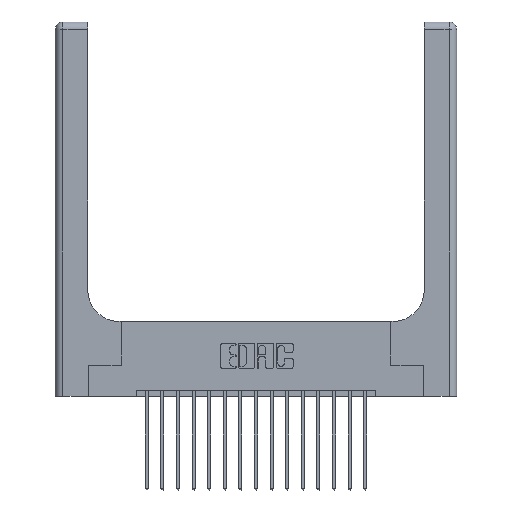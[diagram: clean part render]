
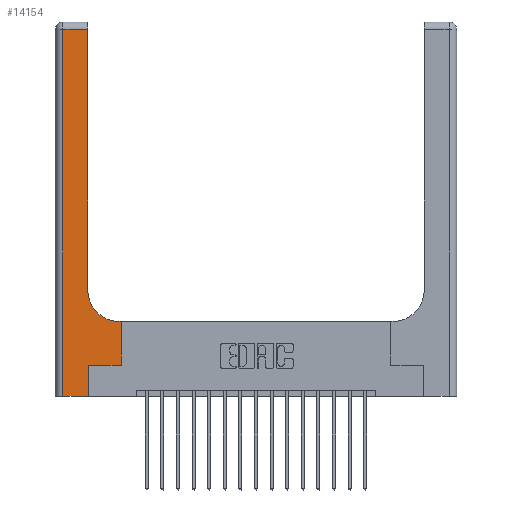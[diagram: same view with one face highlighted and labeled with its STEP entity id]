
A CAD part, top view. The second image highlights one B-rep face of the part: STEP entity #14154.
In plain terms, the highlighted planar face has unit normal (0, 0, 1).
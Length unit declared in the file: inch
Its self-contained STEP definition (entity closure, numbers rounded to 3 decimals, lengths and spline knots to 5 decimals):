
#141 = LINE ( 'NONE', #2446, #17210 ) ;
#380 = PLANE ( 'NONE',  #745 ) ;
#745 = AXIS2_PLACEMENT_3D ( 'NONE', #10289, #16165, #10420 ) ;
#1096 = VECTOR ( 'NONE', #14397, 39.37008 ) ;
#2202 = ORIENTED_EDGE ( 'NONE', *, *, #16690, .T. ) ;
#2215 = LINE ( 'NONE', #14594, #1096 ) ;
#2264 = EDGE_CURVE ( 'NONE', #12493, #14956, #2215, .T. ) ;
#2284 = VECTOR ( 'NONE', #2603, 39.37008 ) ;
#2409 = CARTESIAN_POINT ( 'NONE',  ( 0., 0., 0.37 ) ) ;
#2446 = CARTESIAN_POINT ( 'NONE',  ( 0.26, 0.6, 0.37 ) ) ;
#2603 = DIRECTION ( 'NONE',  ( -1., 0., 0. ) ) ;
#2805 = CARTESIAN_POINT ( 'NONE',  ( 0.26, 0.85, 0.37 ) ) ;
#2861 = DIRECTION ( 'NONE',  ( 0., 1., 0. ) ) ;
#3037 = FACE_OUTER_BOUND ( 'NONE', #11955, .T. ) ;
#3097 = VERTEX_POINT ( 'NONE', #7865 ) ;
#3515 = ORIENTED_EDGE ( 'NONE', *, *, #9226, .T. ) ;
#3967 = ORIENTED_EDGE ( 'NONE', *, *, #6603, .T. ) ;
#4259 = AXIS2_PLACEMENT_3D ( 'NONE', #14259, #14313, #7053 ) ;
#4335 = CARTESIAN_POINT ( 'NONE',  ( 0.26, 2.94, 0.37 ) ) ;
#4403 = EDGE_CURVE ( 'NONE', #17549, #9042, #141, .T. ) ;
#4453 = VECTOR ( 'NONE', #12432, 39.37008 ) ;
#5555 = CARTESIAN_POINT ( 'NONE',  ( 0.265, 0.25, 0.37 ) ) ;
#5765 = CARTESIAN_POINT ( 'NONE',  ( 0.528, 0.25, 0.37 ) ) ;
#5900 = LINE ( 'NONE', #5555, #12452 ) ;
#6108 = CARTESIAN_POINT ( 'NONE',  ( 0.528, 0.6, 0.37 ) ) ;
#6168 = CARTESIAN_POINT ( 'NONE',  ( 0.265, 0., 0.37 ) ) ;
#6223 = DIRECTION ( 'NONE',  ( 0., 1., 0. ) ) ;
#6239 = CARTESIAN_POINT ( 'NONE',  ( 0.51, 0.6, 0.37 ) ) ;
#6603 = EDGE_CURVE ( 'NONE', #14833, #12563, #5900, .T. ) ;
#6992 = VECTOR ( 'NONE', #11159, 39.37008 ) ;
#7053 = DIRECTION ( 'NONE',  ( 1., 0., 0. ) ) ;
#7149 = EDGE_CURVE ( 'NONE', #15370, #12493, #7422, .T. ) ;
#7182 = ORIENTED_EDGE ( 'NONE', *, *, #4403, .T. ) ;
#7422 = LINE ( 'NONE', #12690, #2284 ) ;
#7865 = CARTESIAN_POINT ( 'NONE',  ( 0.265, 0., 0.37 ) ) ;
#7902 = LINE ( 'NONE', #12637, #6992 ) ;
#8383 = VECTOR ( 'NONE', #2861, 39.37008 ) ;
#9042 = VERTEX_POINT ( 'NONE', #6239 ) ;
#9226 = EDGE_CURVE ( 'NONE', #9042, #9868, #12457, .T. ) ;
#9613 = ORIENTED_EDGE ( 'NONE', *, *, #2264, .T. ) ;
#9868 = VERTEX_POINT ( 'NONE', #2805 ) ;
#10289 = CARTESIAN_POINT ( 'NONE',  ( 0., 3., 0.37 ) ) ;
#10420 = DIRECTION ( 'NONE',  ( -1., 0., 0. ) ) ;
#11019 = ORIENTED_EDGE ( 'NONE', *, *, #13062, .T. ) ;
#11134 = EDGE_CURVE ( 'NONE', #14956, #3097, #11226, .T. ) ;
#11159 = DIRECTION ( 'NONE',  ( 0., 1., 0. ) ) ;
#11226 = LINE ( 'NONE', #2409, #4453 ) ;
#11955 = EDGE_LOOP ( 'NONE', ( #14128, #17235, #9613, #18597, #11019, #3967, #2202, #7182, #3515 ) ) ;
#12069 = CARTESIAN_POINT ( 'NONE',  ( 0.528, 0.25, 0.37 ) ) ;
#12093 = VECTOR ( 'NONE', #6223, 39.37008 ) ;
#12168 = CARTESIAN_POINT ( 'NONE',  ( 0.06, 2.94, 0.37 ) ) ;
#12432 = DIRECTION ( 'NONE',  ( 1., 0., 0. ) ) ;
#12452 = VECTOR ( 'NONE', #16348, 39.37008 ) ;
#12457 = CIRCLE ( 'NONE', #4259, 0.25 ) ;
#12493 = VERTEX_POINT ( 'NONE', #12168 ) ;
#12563 = VERTEX_POINT ( 'NONE', #12069 ) ;
#12637 = CARTESIAN_POINT ( 'NONE',  ( 0.26, 3., 0.37 ) ) ;
#12690 = CARTESIAN_POINT ( 'NONE',  ( 0., 2.94, 0.37 ) ) ;
#13062 = EDGE_CURVE ( 'NONE', #3097, #14833, #15246, .T. ) ;
#13718 = DIRECTION ( 'NONE',  ( -1., 0., 0. ) ) ;
#14128 = ORIENTED_EDGE ( 'NONE', *, *, #17308, .T. ) ;
#14154 = ADVANCED_FACE ( 'NONE', ( #3037 ), #380, .F. ) ;
#14259 = CARTESIAN_POINT ( 'NONE',  ( 0.51, 0.85, 0.37 ) ) ;
#14313 = DIRECTION ( 'NONE',  ( 0., 0., -1. ) ) ;
#14397 = DIRECTION ( 'NONE',  ( 0., -1., 0. ) ) ;
#14594 = CARTESIAN_POINT ( 'NONE',  ( 0.06, 3., 0.37 ) ) ;
#14833 = VERTEX_POINT ( 'NONE', #17130 ) ;
#14956 = VERTEX_POINT ( 'NONE', #15808 ) ;
#15246 = LINE ( 'NONE', #6168, #12093 ) ;
#15370 = VERTEX_POINT ( 'NONE', #4335 ) ;
#15808 = CARTESIAN_POINT ( 'NONE',  ( 0.06, 0., 0.37 ) ) ;
#16165 = DIRECTION ( 'NONE',  ( 0., 0., -1. ) ) ;
#16348 = DIRECTION ( 'NONE',  ( 1., 0., 0. ) ) ;
#16690 = EDGE_CURVE ( 'NONE', #12563, #17549, #18558, .T. ) ;
#17130 = CARTESIAN_POINT ( 'NONE',  ( 0.265, 0.25, 0.37 ) ) ;
#17210 = VECTOR ( 'NONE', #13718, 39.37008 ) ;
#17235 = ORIENTED_EDGE ( 'NONE', *, *, #7149, .T. ) ;
#17308 = EDGE_CURVE ( 'NONE', #9868, #15370, #7902, .T. ) ;
#17549 = VERTEX_POINT ( 'NONE', #6108 ) ;
#18558 = LINE ( 'NONE', #5765, #8383 ) ;
#18597 = ORIENTED_EDGE ( 'NONE', *, *, #11134, .T. ) ;
